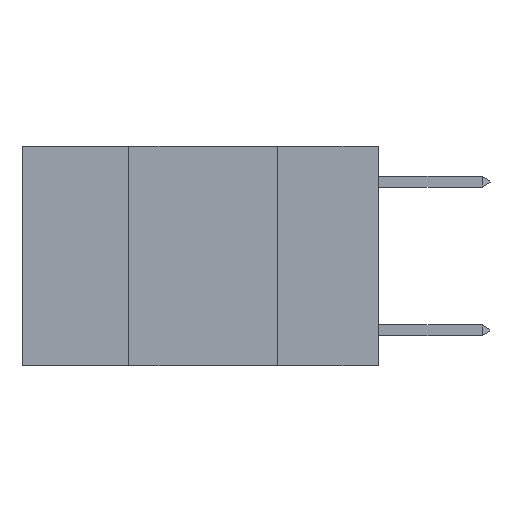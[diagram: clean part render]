
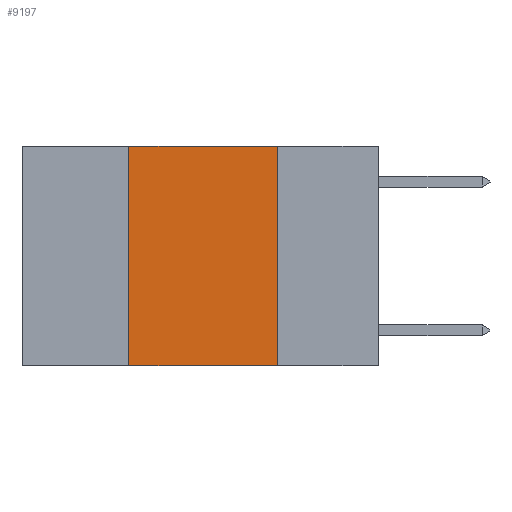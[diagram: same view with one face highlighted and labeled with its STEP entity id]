
A CAD part, left-side view. The second image highlights one B-rep face of the part: STEP entity #9197.
In plain terms, the highlighted planar face has unit normal (-1, 0, 0).
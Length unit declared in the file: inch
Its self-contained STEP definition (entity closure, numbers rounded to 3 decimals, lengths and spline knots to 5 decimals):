
#12 = AXIS2_PLACEMENT_3D ( 'NONE', #3458, #58, #5929 ) ;
#58 = DIRECTION ( 'NONE',  ( 1., 0., 0. ) ) ;
#1154 = EDGE_CURVE ( 'NONE', #6649, #8483, #3087, .T. ) ;
#1734 = ORIENTED_EDGE ( 'NONE', *, *, #1154, .F. ) ;
#2184 = LINE ( 'NONE', #3922, #3891 ) ;
#2528 = LINE ( 'NONE', #9724, #6899 ) ;
#2816 = VECTOR ( 'NONE', #10265, 39.37008 ) ;
#3087 = LINE ( 'NONE', #3732, #2816 ) ;
#3251 = DIRECTION ( 'NONE',  ( 0., -1., 0. ) ) ;
#3458 = CARTESIAN_POINT ( 'NONE',  ( 0., 0.6, 0. ) ) ;
#3494 = CARTESIAN_POINT ( 'NONE',  ( 0., 0.42, -0.37 ) ) ;
#3732 = CARTESIAN_POINT ( 'NONE',  ( 0., 0.17, 0. ) ) ;
#3891 = VECTOR ( 'NONE', #4744, 39.37008 ) ;
#3922 = CARTESIAN_POINT ( 'NONE',  ( 0., 0.42, 0. ) ) ;
#3965 = ORIENTED_EDGE ( 'NONE', *, *, #7281, .F. ) ;
#4302 = DIRECTION ( 'NONE',  ( 0., -1., 0. ) ) ;
#4744 = DIRECTION ( 'NONE',  ( 0., 0., 1. ) ) ;
#5120 = PLANE ( 'NONE',  #12 ) ;
#5685 = EDGE_CURVE ( 'NONE', #9211, #9542, #2184, .T. ) ;
#5929 = DIRECTION ( 'NONE',  ( 0., 0., -1. ) ) ;
#6649 = VERTEX_POINT ( 'NONE', #9287 ) ;
#6899 = VECTOR ( 'NONE', #3251, 39.37008 ) ;
#7281 = EDGE_CURVE ( 'NONE', #9542, #6649, #2528, .T. ) ;
#8344 = CARTESIAN_POINT ( 'NONE',  ( 0., 0.6, -0.37 ) ) ;
#8379 = LINE ( 'NONE', #8344, #10410 ) ;
#8483 = VERTEX_POINT ( 'NONE', #9755 ) ;
#8614 = FACE_OUTER_BOUND ( 'NONE', #9842, .T. ) ;
#9188 = EDGE_CURVE ( 'NONE', #9211, #8483, #8379, .T. ) ;
#9197 = ADVANCED_FACE ( 'NONE', ( #8614 ), #5120, .F. ) ;
#9211 = VERTEX_POINT ( 'NONE', #3494 ) ;
#9287 = CARTESIAN_POINT ( 'NONE',  ( 0., 0.17, 0. ) ) ;
#9542 = VERTEX_POINT ( 'NONE', #9569 ) ;
#9569 = CARTESIAN_POINT ( 'NONE',  ( 0., 0.42, 0. ) ) ;
#9724 = CARTESIAN_POINT ( 'NONE',  ( 0., 0.6, 0. ) ) ;
#9755 = CARTESIAN_POINT ( 'NONE',  ( 0., 0.17, -0.37 ) ) ;
#9842 = EDGE_LOOP ( 'NONE', ( #1734, #3965, #10325, #10565 ) ) ;
#10265 = DIRECTION ( 'NONE',  ( 0., 0., -1. ) ) ;
#10325 = ORIENTED_EDGE ( 'NONE', *, *, #5685, .F. ) ;
#10410 = VECTOR ( 'NONE', #4302, 39.37008 ) ;
#10565 = ORIENTED_EDGE ( 'NONE', *, *, #9188, .T. ) ;
